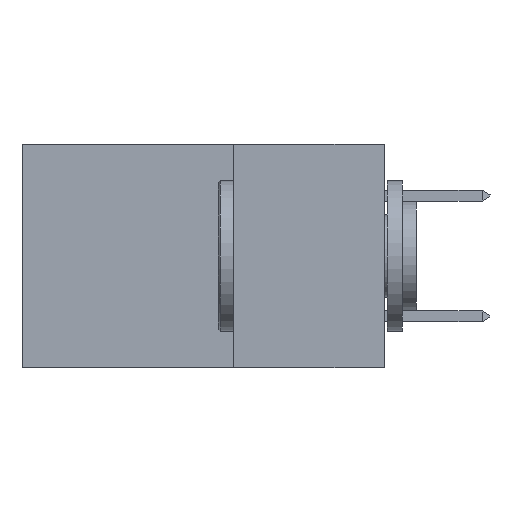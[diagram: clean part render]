
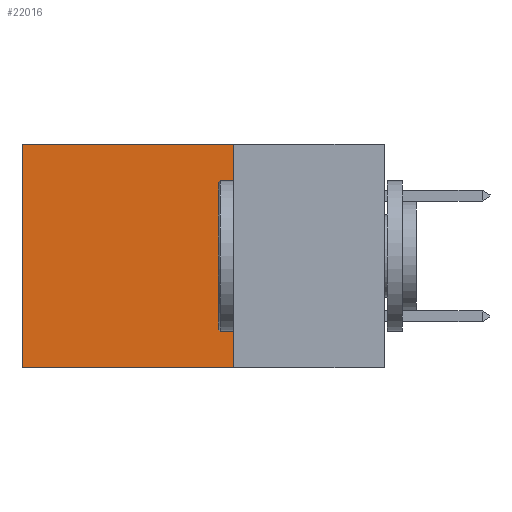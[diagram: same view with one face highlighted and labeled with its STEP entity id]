
A CAD part, left-side view. The second image highlights one B-rep face of the part: STEP entity #22016.
In plain terms, the highlighted planar face has unit normal (-1, 0, 0).
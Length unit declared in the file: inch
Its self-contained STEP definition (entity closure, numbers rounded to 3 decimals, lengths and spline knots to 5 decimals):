
#881 = LINE ( 'NONE', #15377, #17436 ) ;
#1014 = EDGE_CURVE ( 'NONE', #26847, #14408, #881, .T. ) ;
#1465 = AXIS2_PLACEMENT_3D ( 'NONE', #28603, #15723, #25828 ) ;
#1786 = VECTOR ( 'NONE', #13423, 39.37008 ) ;
#2099 = ORIENTED_EDGE ( 'NONE', *, *, #7067, .T. ) ;
#2301 = LINE ( 'NONE', #32374, #12650 ) ;
#2529 = CARTESIAN_POINT ( 'NONE',  ( 0.2875, 0.6, 0. ) ) ;
#2973 = VECTOR ( 'NONE', #20640, 39.37008 ) ;
#3061 = EDGE_CURVE ( 'NONE', #14476, #14408, #17518, .T. ) ;
#3803 = LINE ( 'NONE', #20883, #2973 ) ;
#6826 = VERTEX_POINT ( 'NONE', #31186 ) ;
#7067 = EDGE_CURVE ( 'NONE', #6826, #26847, #3803, .T. ) ;
#10341 = EDGE_LOOP ( 'NONE', ( #19753, #17522, #32224, #2099 ) ) ;
#12650 = VECTOR ( 'NONE', #16437, 39.37008 ) ;
#13423 = DIRECTION ( 'NONE',  ( 0., 1., 0. ) ) ;
#14408 = VERTEX_POINT ( 'NONE', #31055 ) ;
#14476 = VERTEX_POINT ( 'NONE', #28711 ) ;
#15377 = CARTESIAN_POINT ( 'NONE',  ( 0.2875, 0.6, 0. ) ) ;
#15723 = DIRECTION ( 'NONE',  ( 1., 0., 0. ) ) ;
#16437 = DIRECTION ( 'NONE',  ( 0., 0., -1. ) ) ;
#17436 = VECTOR ( 'NONE', #26628, 39.37008 ) ;
#17518 = LINE ( 'NONE', #29924, #1786 ) ;
#17522 = ORIENTED_EDGE ( 'NONE', *, *, #3061, .F. ) ;
#19622 = FACE_OUTER_BOUND ( 'NONE', #10341, .T. ) ;
#19753 = ORIENTED_EDGE ( 'NONE', *, *, #1014, .T. ) ;
#20245 = EDGE_CURVE ( 'NONE', #6826, #14476, #2301, .T. ) ;
#20640 = DIRECTION ( 'NONE',  ( 0., 1., 0. ) ) ;
#20883 = CARTESIAN_POINT ( 'NONE',  ( 0.2875, 0.25, 0. ) ) ;
#22016 = ADVANCED_FACE ( 'NONE', ( #19622 ), #33895, .F. ) ;
#25828 = DIRECTION ( 'NONE',  ( 0., 0., -1. ) ) ;
#26628 = DIRECTION ( 'NONE',  ( 0., 0., -1. ) ) ;
#26847 = VERTEX_POINT ( 'NONE', #2529 ) ;
#28603 = CARTESIAN_POINT ( 'NONE',  ( 0.2875, 0.25, 0. ) ) ;
#28711 = CARTESIAN_POINT ( 'NONE',  ( 0.2875, 0.25, -0.37 ) ) ;
#29924 = CARTESIAN_POINT ( 'NONE',  ( 0.2875, 0.25, -0.37 ) ) ;
#31055 = CARTESIAN_POINT ( 'NONE',  ( 0.2875, 0.6, -0.37 ) ) ;
#31186 = CARTESIAN_POINT ( 'NONE',  ( 0.2875, 0.25, 0. ) ) ;
#32224 = ORIENTED_EDGE ( 'NONE', *, *, #20245, .F. ) ;
#32374 = CARTESIAN_POINT ( 'NONE',  ( 0.2875, 0.25, 0. ) ) ;
#33895 = PLANE ( 'NONE',  #1465 ) ;
